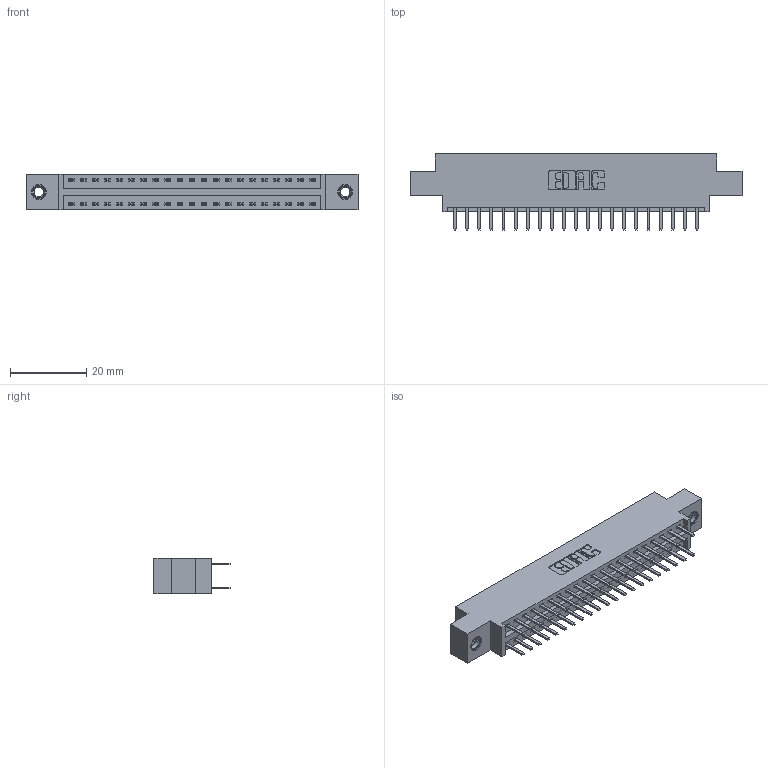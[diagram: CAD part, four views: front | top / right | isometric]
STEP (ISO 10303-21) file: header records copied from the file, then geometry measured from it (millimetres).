
FILE_DESCRIPTION (( 'STEP AP203' ), '1' );
FILE_NAME ('396-042-520-807.STEP', '2018-09-06T23:28:45', ( '' ), ( '' ), 'SwSTEP 2.0', 'SolidWorks 2016', '' );
FILE_SCHEMA (( 'CONFIG_CONTROL_DESIGN' ));
Length unit declared in the file: inch
Products named in the file (4): 345-292-001_345-293-120; 345-250-001_345-250-005-103; 396-042-520-807; 346 Part_0.170 Offset - 0.156 Dia-TI
Assembly tree (45 placements, depth 2):
  396-042-520-807
    346 Part_0.170 Offset - 0.156 Dia-TI
    345-292-001_345-293-120  x42
    345-250-001_345-250-005-103  x2
Bounding box: 87.25 x 20.02 x 9.4 mm (x, y, z)
Volume: 8158.2 mm3; surface area: 11054 mm2
Topology: 45 solids, 45 shells, 2538 faces, 7323 edges, 4762 vertices
Faces by surface type: plane 1666, cylinder 856, cone 12, torus 4
Entity records: 17964 total; most frequent: CARTESIAN_POINT 2987, ORIENTED_EDGE 2902, DIRECTION 2697, EDGE_CURVE 1451, VECTOR 1211, LINE 1211, VERTEX_POINT 960, AXIS2_PLACEMENT_3D 743
